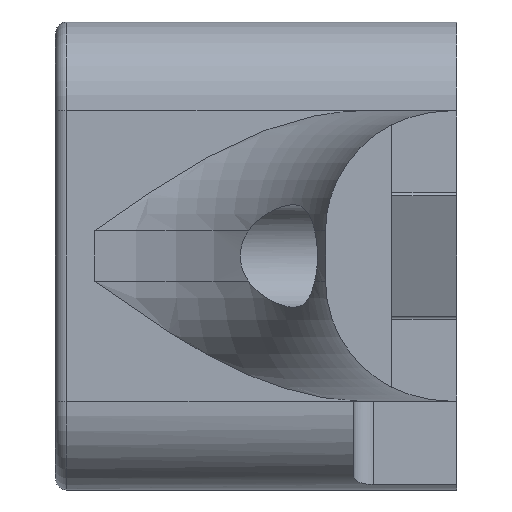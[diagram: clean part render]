
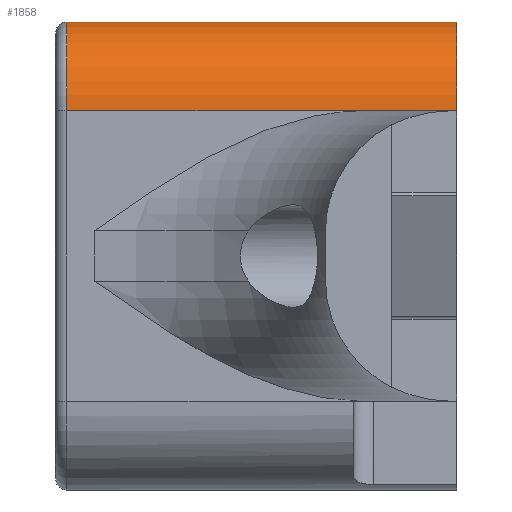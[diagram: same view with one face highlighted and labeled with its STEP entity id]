
A CAD part, front view. The second image highlights one B-rep face of the part: STEP entity #1858.
In plain terms, the highlighted cylindrical face has radius 7.057 mm (diameter 14.114 mm), a partial arc.
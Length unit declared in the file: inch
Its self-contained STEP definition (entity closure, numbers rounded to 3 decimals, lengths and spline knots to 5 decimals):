
#87=CYLINDRICAL_SURFACE('',#2025,0.27784);
#262=FACE_OUTER_BOUND('',#387,.T.);
#387=EDGE_LOOP('',(#1324,#1325,#1326,#1327,#1328));
#515=CIRCLE('',#1981,0.27784);
#545=CIRCLE('',#2020,0.27784);
#645=LINE('',#2822,#714);
#646=LINE('',#2823,#715);
#647=LINE('',#2824,#716);
#714=VECTOR('',#2301,0.92403);
#715=VECTOR('',#2302,0.29397);
#716=VECTOR('',#2303,1.218);
#772=VERTEX_POINT('',#2676);
#773=VERTEX_POINT('',#2678);
#809=VERTEX_POINT('',#2803);
#811=VERTEX_POINT('',#2811);
#813=VERTEX_POINT('',#2821);
#969=EDGE_CURVE('',#773,#772,#515,.T.);
#1014=EDGE_CURVE('',#809,#811,#545,.T.);
#1018=EDGE_CURVE('',#809,#813,#645,.T.);
#1019=EDGE_CURVE('',#773,#813,#646,.T.);
#1020=EDGE_CURVE('',#772,#811,#647,.T.);
#1324=ORIENTED_EDGE('',*,*,#1014,.F.);
#1325=ORIENTED_EDGE('',*,*,#1018,.T.);
#1326=ORIENTED_EDGE('',*,*,#1019,.F.);
#1327=ORIENTED_EDGE('',*,*,#969,.T.);
#1328=ORIENTED_EDGE('',*,*,#1020,.T.);
#1858=ADVANCED_FACE('',(#262),#87,.T.);
#1981=AXIS2_PLACEMENT_3D('',#2679,#2197,#2198);
#2020=AXIS2_PLACEMENT_3D('',#2813,#2288,#2289);
#2025=AXIS2_PLACEMENT_3D('',#2820,#2299,#2300);
#2197=DIRECTION('center_axis',(-1.,0.,0.));
#2198=DIRECTION('ref_axis',(0.,0.,1.));
#2288=DIRECTION('center_axis',(-1.,0.,0.));
#2289=DIRECTION('ref_axis',(0.,1.,0.));
#2299=DIRECTION('center_axis',(-1.,0.,0.));
#2300=DIRECTION('ref_axis',(0.,0.,1.));
#2301=DIRECTION('',(1.,0.,0.));
#2302=DIRECTION('',(-1.,0.,0.));
#2303=DIRECTION('',(-1.,0.,0.));
#2676=CARTESIAN_POINT('',(-6.25,-0.22666,0.73097));
#2678=CARTESIAN_POINT('',(-6.25,-0.5045,0.45313));
#2679=CARTESIAN_POINT('Origin',(-6.25,-0.22666,0.45313));
#2803=CARTESIAN_POINT('',(-7.468,-0.5045,0.45313));
#2811=CARTESIAN_POINT('',(-7.468,-0.22666,0.73097));
#2813=CARTESIAN_POINT('Origin',(-7.468,-0.22666,0.45313));
#2820=CARTESIAN_POINT('Origin',(-0.84663,-0.22666,0.45313));
#2821=CARTESIAN_POINT('',(-6.54397,-0.5045,0.45313));
#2822=CARTESIAN_POINT('',(-7.468,-0.5045,0.45313));
#2823=CARTESIAN_POINT('',(-6.25,-0.5045,0.45313));
#2824=CARTESIAN_POINT('',(-6.25,-0.22666,0.73097));
